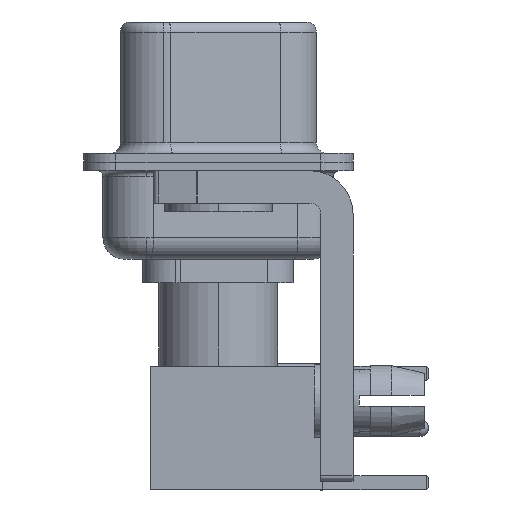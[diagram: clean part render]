
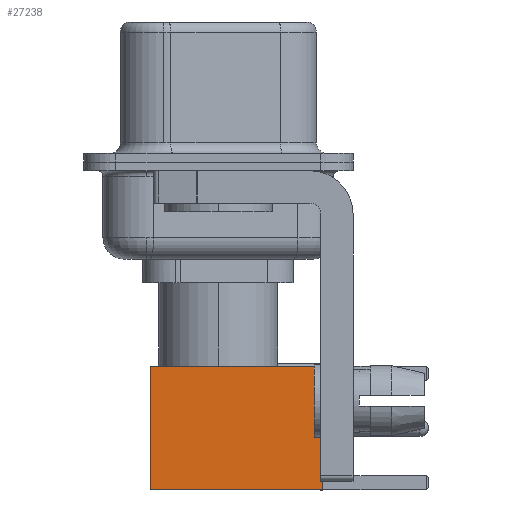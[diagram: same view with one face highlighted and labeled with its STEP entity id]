
A CAD part, left-side view. The second image highlights one B-rep face of the part: STEP entity #27238.
In plain terms, the highlighted face is planar.
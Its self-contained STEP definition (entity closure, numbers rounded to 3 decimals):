
#662 = CARTESIAN_POINT ( 'NONE',  ( -2.875, 2.875, 8. ) ) ;
#1913 = PLANE ( 'NONE',  #8228 ) ;
#2013 = DIRECTION ( 'NONE',  ( -1., 0., 0. ) ) ;
#4751 = CARTESIAN_POINT ( 'NONE',  ( 0., 2.875, 8. ) ) ;
#4964 = CARTESIAN_POINT ( 'NONE',  ( 0., 2.875, 0. ) ) ;
#5891 = EDGE_CURVE ( 'NONE', #23477, #25180, #30340, .T. ) ;
#7018 = DIRECTION ( 'NONE',  ( 0., 0., -1. ) ) ;
#7871 = CARTESIAN_POINT ( 'NONE',  ( -2.875, 2.875, 0. ) ) ;
#8228 = AXIS2_PLACEMENT_3D ( 'NONE', #21922, #18985, #14685 ) ;
#9240 = EDGE_CURVE ( 'NONE', #21563, #28019, #19477, .T. ) ;
#10115 = VECTOR ( 'NONE', #29038, 1000. ) ;
#11135 = ORIENTED_EDGE ( 'NONE', *, *, #5891, .F. ) ;
#13567 = EDGE_CURVE ( 'NONE', #21563, #23477, #26880, .T. ) ;
#14140 = VECTOR ( 'NONE', #2013, 1000. ) ;
#14460 = LINE ( 'NONE', #4964, #14140 ) ;
#14685 = DIRECTION ( 'NONE',  ( 0., 0., 1. ) ) ;
#17218 = VECTOR ( 'NONE', #7018, 1000. ) ;
#18531 = CARTESIAN_POINT ( 'NONE',  ( -2.875, 2.875, 0. ) ) ;
#18743 = EDGE_CURVE ( 'NONE', #28019, #25180, #14460, .T. ) ;
#18985 = DIRECTION ( 'NONE',  ( 0., 1., 0. ) ) ;
#19271 = VECTOR ( 'NONE', #25733, 1000. ) ;
#19477 = LINE ( 'NONE', #29486, #17218 ) ;
#21563 = VERTEX_POINT ( 'NONE', #31721 ) ;
#21922 = CARTESIAN_POINT ( 'NONE',  ( 2.875, 2.875, 0. ) ) ;
#23014 = EDGE_LOOP ( 'NONE', ( #31799, #27514, #11135, #29758 ) ) ;
#23477 = VERTEX_POINT ( 'NONE', #662 ) ;
#25180 = VERTEX_POINT ( 'NONE', #18531 ) ;
#25733 = DIRECTION ( 'NONE',  ( 0., 0., -1. ) ) ;
#26404 = CARTESIAN_POINT ( 'NONE',  ( 2.875, 2.875, 0. ) ) ;
#26880 = LINE ( 'NONE', #4751, #10115 ) ;
#27238 = ADVANCED_FACE ( 'NONE', ( #29304 ), #1913, .T. ) ;
#27514 = ORIENTED_EDGE ( 'NONE', *, *, #18743, .T. ) ;
#28019 = VERTEX_POINT ( 'NONE', #26404 ) ;
#29038 = DIRECTION ( 'NONE',  ( -1., 0., 0. ) ) ;
#29304 = FACE_OUTER_BOUND ( 'NONE', #23014, .T. ) ;
#29486 = CARTESIAN_POINT ( 'NONE',  ( 2.875, 2.875, 0. ) ) ;
#29758 = ORIENTED_EDGE ( 'NONE', *, *, #13567, .F. ) ;
#30340 = LINE ( 'NONE', #7871, #19271 ) ;
#31721 = CARTESIAN_POINT ( 'NONE',  ( 2.875, 2.875, 8. ) ) ;
#31799 = ORIENTED_EDGE ( 'NONE', *, *, #9240, .T. ) ;
